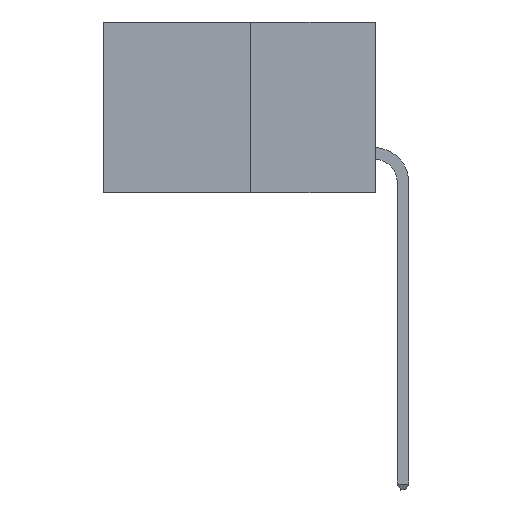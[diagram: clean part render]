
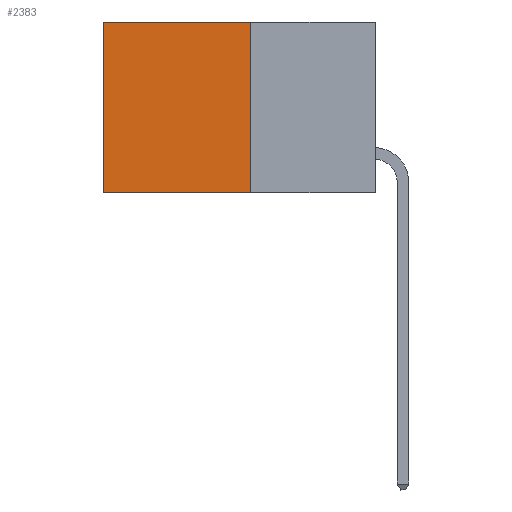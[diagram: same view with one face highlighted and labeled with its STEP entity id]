
A CAD part, left-side view. The second image highlights one B-rep face of the part: STEP entity #2383.
In plain terms, the highlighted planar face has unit normal (-1, 0, 0).
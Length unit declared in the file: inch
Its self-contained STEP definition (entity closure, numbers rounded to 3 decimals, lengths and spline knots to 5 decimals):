
#296 = CARTESIAN_POINT ( 'NONE',  ( 0.277, 0.27, -0.37 ) ) ;
#382 = VERTEX_POINT ( 'NONE', #6590 ) ;
#492 = LINE ( 'NONE', #6434, #2983 ) ;
#502 = CARTESIAN_POINT ( 'NONE',  ( 0.277, 0.27, -0.37 ) ) ;
#505 = VERTEX_POINT ( 'NONE', #11005 ) ;
#863 = ORIENTED_EDGE ( 'NONE', *, *, #5234, .T. ) ;
#1236 = EDGE_CURVE ( 'NONE', #4886, #382, #10879, .T. ) ;
#1273 = DIRECTION ( 'NONE',  ( 1., 0., 0. ) ) ;
#1290 = PLANE ( 'NONE',  #11507 ) ;
#1945 = DIRECTION ( 'NONE',  ( 0., 0., -1. ) ) ;
#2279 = VECTOR ( 'NONE', #5401, 39.37008 ) ;
#2383 = ADVANCED_FACE ( 'NONE', ( #7906 ), #1290, .F. ) ;
#2701 = EDGE_LOOP ( 'NONE', ( #863, #10104, #9037, #9250 ) ) ;
#2822 = LINE ( 'NONE', #296, #5267 ) ;
#2983 = VECTOR ( 'NONE', #8272, 39.37008 ) ;
#3546 = EDGE_CURVE ( 'NONE', #505, #6493, #4446, .T. ) ;
#3707 = VECTOR ( 'NONE', #5164, 39.37008 ) ;
#4446 = LINE ( 'NONE', #5752, #2279 ) ;
#4886 = VERTEX_POINT ( 'NONE', #10417 ) ;
#5164 = DIRECTION ( 'NONE',  ( 0., 1., 0. ) ) ;
#5234 = EDGE_CURVE ( 'NONE', #6493, #382, #492, .T. ) ;
#5267 = VECTOR ( 'NONE', #9458, 39.37008 ) ;
#5401 = DIRECTION ( 'NONE',  ( 0., 1., 0. ) ) ;
#5487 = EDGE_CURVE ( 'NONE', #505, #4886, #2822, .T. ) ;
#5752 = CARTESIAN_POINT ( 'NONE',  ( 0.277, 0.27, 0. ) ) ;
#6434 = CARTESIAN_POINT ( 'NONE',  ( 0.277, 0.59, -0.37 ) ) ;
#6493 = VERTEX_POINT ( 'NONE', #11693 ) ;
#6590 = CARTESIAN_POINT ( 'NONE',  ( 0.277, 0.59, -0.37 ) ) ;
#7455 = CARTESIAN_POINT ( 'NONE',  ( 0.277, 0.27, -0.37 ) ) ;
#7906 = FACE_OUTER_BOUND ( 'NONE', #2701, .T. ) ;
#8272 = DIRECTION ( 'NONE',  ( 0., 0., -1. ) ) ;
#9037 = ORIENTED_EDGE ( 'NONE', *, *, #5487, .F. ) ;
#9250 = ORIENTED_EDGE ( 'NONE', *, *, #3546, .T. ) ;
#9458 = DIRECTION ( 'NONE',  ( 0., 0., -1. ) ) ;
#10104 = ORIENTED_EDGE ( 'NONE', *, *, #1236, .F. ) ;
#10417 = CARTESIAN_POINT ( 'NONE',  ( 0.277, 0.27, -0.37 ) ) ;
#10879 = LINE ( 'NONE', #7455, #3707 ) ;
#11005 = CARTESIAN_POINT ( 'NONE',  ( 0.277, 0.27, 0. ) ) ;
#11507 = AXIS2_PLACEMENT_3D ( 'NONE', #502, #1273, #1945 ) ;
#11693 = CARTESIAN_POINT ( 'NONE',  ( 0.277, 0.59, 0. ) ) ;
